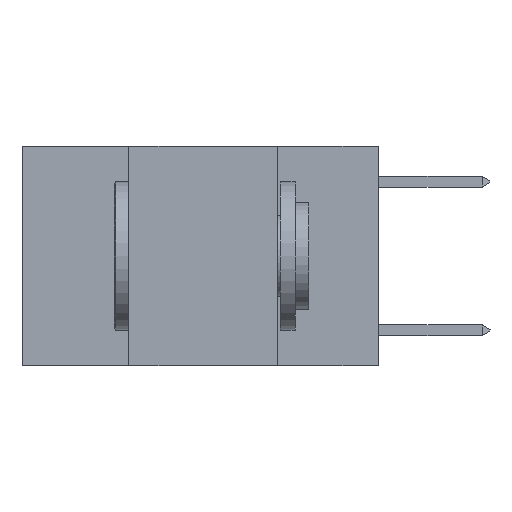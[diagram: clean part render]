
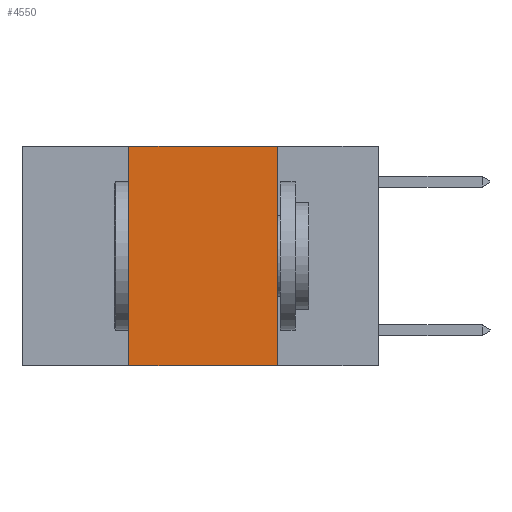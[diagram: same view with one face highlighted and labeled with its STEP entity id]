
A CAD part, left-side view. The second image highlights one B-rep face of the part: STEP entity #4550.
In plain terms, the highlighted planar face has unit normal (-1, 0, 0).
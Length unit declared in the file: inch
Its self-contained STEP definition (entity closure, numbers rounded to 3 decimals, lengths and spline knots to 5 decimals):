
#750 = VECTOR ( 'NONE', #10807, 39.37008 ) ;
#1185 = VERTEX_POINT ( 'NONE', #5799 ) ;
#2274 = CARTESIAN_POINT ( 'NONE',  ( 0., 0.42, 0. ) ) ;
#3885 = FACE_OUTER_BOUND ( 'NONE', #6914, .T. ) ;
#4381 = VECTOR ( 'NONE', #11042, 39.37008 ) ;
#4550 = ADVANCED_FACE ( 'NONE', ( #3885 ), #6571, .F. ) ;
#4926 = LINE ( 'NONE', #13236, #5568 ) ;
#5062 = CARTESIAN_POINT ( 'NONE',  ( 0., 0.42, -0.37 ) ) ;
#5568 = VECTOR ( 'NONE', #9468, 39.37008 ) ;
#5799 = CARTESIAN_POINT ( 'NONE',  ( 0., 0.17, -0.37 ) ) ;
#6373 = VERTEX_POINT ( 'NONE', #15002 ) ;
#6571 = PLANE ( 'NONE',  #8673 ) ;
#6646 = LINE ( 'NONE', #2274, #750 ) ;
#6832 = CARTESIAN_POINT ( 'NONE',  ( 0., 0.6, 0. ) ) ;
#6914 = EDGE_LOOP ( 'NONE', ( #18061, #16808, #9053, #10530 ) ) ;
#8673 = AXIS2_PLACEMENT_3D ( 'NONE', #6832, #16526, #9716 ) ;
#8677 = CARTESIAN_POINT ( 'NONE',  ( 0., 0.6, -0.37 ) ) ;
#9053 = ORIENTED_EDGE ( 'NONE', *, *, #16738, .F. ) ;
#9468 = DIRECTION ( 'NONE',  ( 0., -1., 0. ) ) ;
#9716 = DIRECTION ( 'NONE',  ( 0., 0., -1. ) ) ;
#9757 = CARTESIAN_POINT ( 'NONE',  ( 0., 0.17, 0. ) ) ;
#9890 = LINE ( 'NONE', #8677, #17678 ) ;
#10067 = DIRECTION ( 'NONE',  ( 0., -1., 0. ) ) ;
#10530 = ORIENTED_EDGE ( 'NONE', *, *, #16788, .T. ) ;
#10776 = VERTEX_POINT ( 'NONE', #5062 ) ;
#10807 = DIRECTION ( 'NONE',  ( 0., 0., 1. ) ) ;
#11042 = DIRECTION ( 'NONE',  ( 0., 0., -1. ) ) ;
#11134 = LINE ( 'NONE', #9757, #4381 ) ;
#13236 = CARTESIAN_POINT ( 'NONE',  ( 0., 0.6, 0. ) ) ;
#14557 = CARTESIAN_POINT ( 'NONE',  ( 0., 0.42, 0. ) ) ;
#15002 = CARTESIAN_POINT ( 'NONE',  ( 0., 0.17, 0. ) ) ;
#16519 = VERTEX_POINT ( 'NONE', #14557 ) ;
#16526 = DIRECTION ( 'NONE',  ( 1., 0., 0. ) ) ;
#16738 = EDGE_CURVE ( 'NONE', #10776, #16519, #6646, .T. ) ;
#16788 = EDGE_CURVE ( 'NONE', #10776, #1185, #9890, .T. ) ;
#16808 = ORIENTED_EDGE ( 'NONE', *, *, #18101, .F. ) ;
#17678 = VECTOR ( 'NONE', #10067, 39.37008 ) ;
#17732 = EDGE_CURVE ( 'NONE', #6373, #1185, #11134, .T. ) ;
#18061 = ORIENTED_EDGE ( 'NONE', *, *, #17732, .F. ) ;
#18101 = EDGE_CURVE ( 'NONE', #16519, #6373, #4926, .T. ) ;
